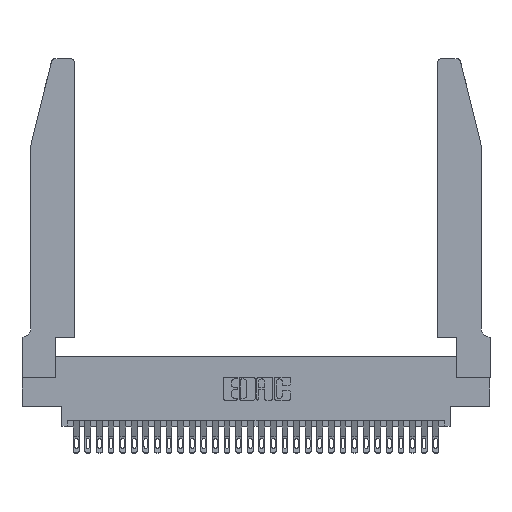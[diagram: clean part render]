
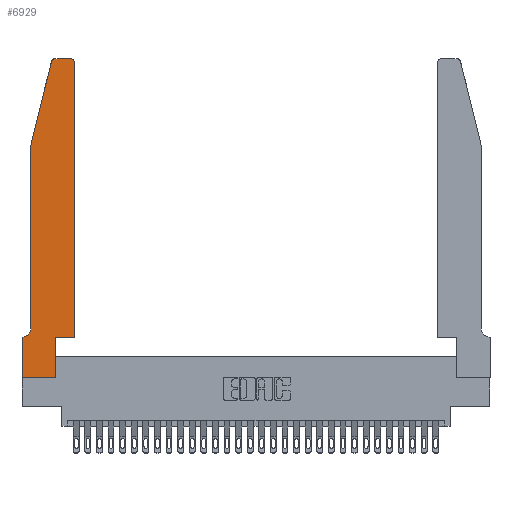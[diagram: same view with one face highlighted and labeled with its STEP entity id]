
A CAD part, top view. The second image highlights one B-rep face of the part: STEP entity #6929.
In plain terms, the highlighted planar face has unit normal (0, 0, 1).
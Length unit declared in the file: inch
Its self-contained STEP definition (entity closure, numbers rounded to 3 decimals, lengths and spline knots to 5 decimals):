
#143 = ORIENTED_EDGE ( 'NONE', *, *, #17775, .T. ) ;
#211 = AXIS2_PLACEMENT_3D ( 'NONE', #28679, #29116, #31078 ) ;
#355 = CARTESIAN_POINT ( 'NONE',  ( 0.0755, 2., 0.37 ) ) ;
#863 = VECTOR ( 'NONE', #5521, 39.37008 ) ;
#1121 = ORIENTED_EDGE ( 'NONE', *, *, #30356, .T. ) ;
#1320 = PLANE ( 'NONE',  #21831 ) ;
#1971 = ORIENTED_EDGE ( 'NONE', *, *, #2189, .T. ) ;
#2189 = EDGE_CURVE ( 'NONE', #25675, #23995, #9609, .T. ) ;
#2291 = VERTEX_POINT ( 'NONE', #27333 ) ;
#2732 = CARTESIAN_POINT ( 'NONE',  ( 0., 0., 0.37 ) ) ;
#2769 = CARTESIAN_POINT ( 'NONE',  ( 0.0055, 0.42, 0.37 ) ) ;
#2865 = DIRECTION ( 'NONE',  ( 0., 0., -1. ) ) ;
#3138 = VECTOR ( 'NONE', #27773, 39.37008 ) ;
#3395 = DIRECTION ( 'NONE',  ( -1., 0., 0. ) ) ;
#3547 = EDGE_CURVE ( 'NONE', #6048, #24187, #5732, .T. ) ;
#3666 = VERTEX_POINT ( 'NONE', #30575 ) ;
#3847 = CARTESIAN_POINT ( 'NONE',  ( 0.2865, 0., 0.37 ) ) ;
#4819 = DIRECTION ( 'NONE',  ( 0., 0., 1. ) ) ;
#4910 = EDGE_CURVE ( 'NONE', #8472, #6048, #21733, .T. ) ;
#5521 = DIRECTION ( 'NONE',  ( 0., -1., 0. ) ) ;
#5616 = EDGE_LOOP ( 'NONE', ( #1121, #1971, #22829, #30449, #11735, #7620, #27179, #29010, #14579, #143, #14950, #17066 ) ) ;
#5732 = CIRCLE ( 'NONE', #13160, 0.07 ) ;
#5906 = CARTESIAN_POINT ( 'NONE',  ( 0.0755, 0.42, 0.37 ) ) ;
#5929 = LINE ( 'NONE', #30608, #17041 ) ;
#6048 = VERTEX_POINT ( 'NONE', #5906 ) ;
#6079 = VECTOR ( 'NONE', #22000, 39.37008 ) ;
#6777 = CARTESIAN_POINT ( 'NONE',  ( 0.0055, 0.35, 0.37 ) ) ;
#6929 = ADVANCED_FACE ( 'NONE', ( #22273 ), #1320, .T. ) ;
#6970 = LINE ( 'NONE', #19799, #19216 ) ;
#7039 = EDGE_CURVE ( 'NONE', #30163, #14650, #23018, .T. ) ;
#7451 = CIRCLE ( 'NONE', #26023, 0.03 ) ;
#7464 = EDGE_CURVE ( 'NONE', #24187, #25469, #28337, .T. ) ;
#7524 = VERTEX_POINT ( 'NONE', #13330 ) ;
#7620 = ORIENTED_EDGE ( 'NONE', *, *, #7464, .T. ) ;
#7659 = CARTESIAN_POINT ( 'NONE',  ( 0., 0.35, 0.37 ) ) ;
#7924 = LINE ( 'NONE', #23073, #26683 ) ;
#8203 = CARTESIAN_POINT ( 'NONE',  ( 0., 0., 0.37 ) ) ;
#8351 = DIRECTION ( 'NONE',  ( 1., 0., 0. ) ) ;
#8472 = VERTEX_POINT ( 'NONE', #12070 ) ;
#9609 = CIRCLE ( 'NONE', #211, 0.03 ) ;
#10923 = DIRECTION ( 'NONE',  ( 0., 0., 1. ) ) ;
#11735 = ORIENTED_EDGE ( 'NONE', *, *, #3547, .T. ) ;
#11949 = DIRECTION ( 'NONE',  ( 1., 0., 0. ) ) ;
#12070 = CARTESIAN_POINT ( 'NONE',  ( 0.0755, 2., 0.37 ) ) ;
#12278 = VECTOR ( 'NONE', #27364, 39.37008 ) ;
#12568 = EDGE_CURVE ( 'NONE', #14650, #7524, #6970, .T. ) ;
#13160 = AXIS2_PLACEMENT_3D ( 'NONE', #2769, #2865, #3395 ) ;
#13330 = CARTESIAN_POINT ( 'NONE',  ( 0.2865, 0.35, 0.37 ) ) ;
#13700 = LINE ( 'NONE', #355, #6079 ) ;
#14165 = DIRECTION ( 'NONE',  ( 0., -1., 0. ) ) ;
#14579 = ORIENTED_EDGE ( 'NONE', *, *, #12568, .T. ) ;
#14650 = VERTEX_POINT ( 'NONE', #3847 ) ;
#14926 = EDGE_CURVE ( 'NONE', #23995, #8472, #13700, .T. ) ;
#14950 = ORIENTED_EDGE ( 'NONE', *, *, #22940, .T. ) ;
#15895 = CARTESIAN_POINT ( 'NONE',  ( 0.284, 2.75, 0.37 ) ) ;
#16151 = DIRECTION ( 'NONE',  ( -1., 0., 0. ) ) ;
#17041 = VECTOR ( 'NONE', #8351, 39.37008 ) ;
#17066 = ORIENTED_EDGE ( 'NONE', *, *, #20389, .T. ) ;
#17340 = DIRECTION ( 'NONE',  ( 0., 1., 0. ) ) ;
#17558 = VECTOR ( 'NONE', #14165, 39.37008 ) ;
#17775 = EDGE_CURVE ( 'NONE', #7524, #2291, #5929, .T. ) ;
#18450 = VECTOR ( 'NONE', #30865, 39.37008 ) ;
#18472 = CARTESIAN_POINT ( 'NONE',  ( 0., 0.35, 0.37 ) ) ;
#18580 = VERTEX_POINT ( 'NONE', #20951 ) ;
#18674 = DIRECTION ( 'NONE',  ( 1., 0., 0. ) ) ;
#18913 = CARTESIAN_POINT ( 'NONE',  ( 0.4505, 0.35, 0.37 ) ) ;
#19216 = VECTOR ( 'NONE', #17340, 39.37008 ) ;
#19799 = CARTESIAN_POINT ( 'NONE',  ( 0.2865, 0.35, 0.37 ) ) ;
#20389 = EDGE_CURVE ( 'NONE', #18580, #3666, #7451, .T. ) ;
#20951 = CARTESIAN_POINT ( 'NONE',  ( 0.4505, 2.72, 0.37 ) ) ;
#21314 = EDGE_CURVE ( 'NONE', #25469, #30163, #26882, .T. ) ;
#21733 = LINE ( 'NONE', #31269, #17558 ) ;
#21831 = AXIS2_PLACEMENT_3D ( 'NONE', #18472, #10923, #18674 ) ;
#22000 = DIRECTION ( 'NONE',  ( -0.239, -0.971, 0. ) ) ;
#22273 = FACE_OUTER_BOUND ( 'NONE', #5616, .T. ) ;
#22829 = ORIENTED_EDGE ( 'NONE', *, *, #14926, .T. ) ;
#22940 = EDGE_CURVE ( 'NONE', #2291, #18580, #30278, .T. ) ;
#23018 = LINE ( 'NONE', #25367, #3138 ) ;
#23073 = CARTESIAN_POINT ( 'NONE',  ( 0.2605, 2.75, 0.37 ) ) ;
#23252 = CARTESIAN_POINT ( 'NONE',  ( 0.25487, 2.72718, 0.37 ) ) ;
#23995 = VERTEX_POINT ( 'NONE', #23252 ) ;
#24187 = VERTEX_POINT ( 'NONE', #6777 ) ;
#25367 = CARTESIAN_POINT ( 'NONE',  ( 0., 0., 0.37 ) ) ;
#25469 = VERTEX_POINT ( 'NONE', #7659 ) ;
#25675 = VERTEX_POINT ( 'NONE', #15895 ) ;
#26023 = AXIS2_PLACEMENT_3D ( 'NONE', #26498, #4819, #11949 ) ;
#26498 = CARTESIAN_POINT ( 'NONE',  ( 0.4205, 2.72, 0.37 ) ) ;
#26683 = VECTOR ( 'NONE', #16151, 39.37008 ) ;
#26882 = LINE ( 'NONE', #2732, #863 ) ;
#27179 = ORIENTED_EDGE ( 'NONE', *, *, #21314, .T. ) ;
#27333 = CARTESIAN_POINT ( 'NONE',  ( 0.4505, 0.35, 0.37 ) ) ;
#27364 = DIRECTION ( 'NONE',  ( -1., 0., 0. ) ) ;
#27773 = DIRECTION ( 'NONE',  ( 1., 0., 0. ) ) ;
#28337 = LINE ( 'NONE', #29296, #12278 ) ;
#28679 = CARTESIAN_POINT ( 'NONE',  ( 0.284, 2.72, 0.37 ) ) ;
#29010 = ORIENTED_EDGE ( 'NONE', *, *, #7039, .T. ) ;
#29116 = DIRECTION ( 'NONE',  ( 0., 0., 1. ) ) ;
#29296 = CARTESIAN_POINT ( 'NONE',  ( 0.0755, 0.35, 0.37 ) ) ;
#30163 = VERTEX_POINT ( 'NONE', #8203 ) ;
#30278 = LINE ( 'NONE', #18913, #18450 ) ;
#30356 = EDGE_CURVE ( 'NONE', #3666, #25675, #7924, .T. ) ;
#30449 = ORIENTED_EDGE ( 'NONE', *, *, #4910, .T. ) ;
#30575 = CARTESIAN_POINT ( 'NONE',  ( 0.4205, 2.75, 0.37 ) ) ;
#30608 = CARTESIAN_POINT ( 'NONE',  ( 0.4505, 0.35, 0.37 ) ) ;
#30865 = DIRECTION ( 'NONE',  ( 0., 1., 0. ) ) ;
#31078 = DIRECTION ( 'NONE',  ( 1., 0., 0. ) ) ;
#31269 = CARTESIAN_POINT ( 'NONE',  ( 0.0755, 2., 0.37 ) ) ;
